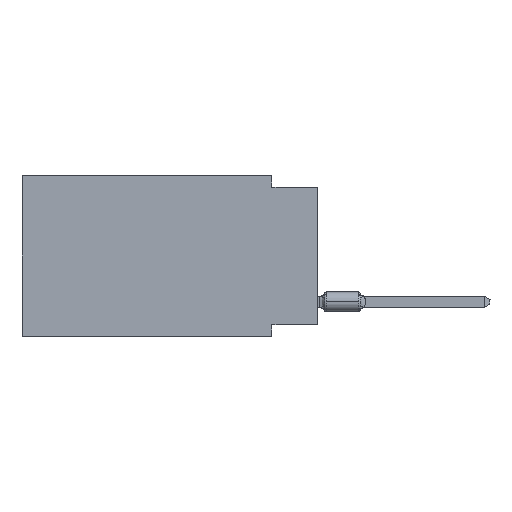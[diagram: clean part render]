
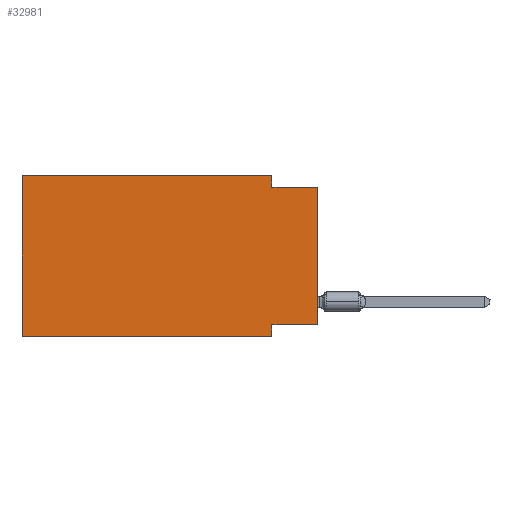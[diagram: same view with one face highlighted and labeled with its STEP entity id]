
A CAD part, left-side view. The second image highlights one B-rep face of the part: STEP entity #32981.
In plain terms, the highlighted planar face has unit normal (-1, 0, 0).
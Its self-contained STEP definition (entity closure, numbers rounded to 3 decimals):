
#937 = DIRECTION ( 'NONE',  ( 0., 0., -1. ) ) ;
#3139 = CARTESIAN_POINT ( 'NONE',  ( 0., 0., 0. ) ) ;
#5009 = DIRECTION ( 'NONE',  ( 0., 0., -1. ) ) ;
#5871 = ORIENTED_EDGE ( 'NONE', *, *, #47507, .F. ) ;
#8277 = EDGE_CURVE ( 'NONE', #50428, #93197, #84382, .T. ) ;
#11157 = ORIENTED_EDGE ( 'NONE', *, *, #21872, .F. ) ;
#12408 = DIRECTION ( 'NONE',  ( 0., 0., -1. ) ) ;
#14637 = DIRECTION ( 'NONE',  ( 0., 1., 0. ) ) ;
#19350 = ORIENTED_EDGE ( 'NONE', *, *, #37590, .F. ) ;
#19694 = DIRECTION ( 'NONE',  ( 0., 0., 1. ) ) ;
#21663 = CARTESIAN_POINT ( 'NONE',  ( 0., 2.54, -8.255 ) ) ;
#21872 = EDGE_CURVE ( 'NONE', #93706, #64156, #83534, .T. ) ;
#22099 = CARTESIAN_POINT ( 'NONE',  ( 0., 2.54, 0. ) ) ;
#23579 = CARTESIAN_POINT ( 'NONE',  ( 0., 16.383, 0. ) ) ;
#24098 = LINE ( 'NONE', #56725, #70165 ) ;
#24640 = CARTESIAN_POINT ( 'NONE',  ( 0., 16.383, -8.89 ) ) ;
#24644 = EDGE_CURVE ( 'NONE', #91051, #93197, #24098, .T. ) ;
#25724 = VECTOR ( 'NONE', #14637, 1000. ) ;
#25810 = EDGE_CURVE ( 'NONE', #64417, #26531, #81307, .T. ) ;
#26531 = VERTEX_POINT ( 'NONE', #54907 ) ;
#27731 = VECTOR ( 'NONE', #87739, 1000. ) ;
#29059 = LINE ( 'NONE', #22099, #90277 ) ;
#31753 = CARTESIAN_POINT ( 'NONE',  ( 0., 0., -8.255 ) ) ;
#32981 = ADVANCED_FACE ( 'NONE', ( #86282 ), #53676, .F. ) ;
#34753 = VERTEX_POINT ( 'NONE', #58322 ) ;
#37590 = EDGE_CURVE ( 'NONE', #50428, #93706, #55281, .T. ) ;
#40272 = VECTOR ( 'NONE', #19694, 1000. ) ;
#44098 = DIRECTION ( 'NONE',  ( 1., 0., 0. ) ) ;
#44999 = EDGE_CURVE ( 'NONE', #26531, #34753, #105078, .T. ) ;
#45669 = CARTESIAN_POINT ( 'NONE',  ( 0., 16.383, 0. ) ) ;
#46533 = CARTESIAN_POINT ( 'NONE',  ( 0., 2.54, -8.89 ) ) ;
#47507 = EDGE_CURVE ( 'NONE', #34753, #91051, #29059, .T. ) ;
#49177 = VECTOR ( 'NONE', #12408, 1000. ) ;
#50428 = VERTEX_POINT ( 'NONE', #71723 ) ;
#53676 = PLANE ( 'NONE',  #61185 ) ;
#54407 = CARTESIAN_POINT ( 'NONE',  ( 0., 0., -0.635 ) ) ;
#54907 = CARTESIAN_POINT ( 'NONE',  ( 0., 16.383, 0. ) ) ;
#55112 = EDGE_CURVE ( 'NONE', #64417, #64156, #89337, .T. ) ;
#55281 = LINE ( 'NONE', #31753, #25724 ) ;
#56725 = CARTESIAN_POINT ( 'NONE',  ( 0., 0., -0.635 ) ) ;
#58322 = CARTESIAN_POINT ( 'NONE',  ( 0., 2.54, 0. ) ) ;
#61089 = CARTESIAN_POINT ( 'NONE',  ( 0., 2.54, -0.635 ) ) ;
#61185 = AXIS2_PLACEMENT_3D ( 'NONE', #45669, #44098, #937 ) ;
#63545 = ORIENTED_EDGE ( 'NONE', *, *, #25810, .F. ) ;
#64156 = VERTEX_POINT ( 'NONE', #46533 ) ;
#64417 = VERTEX_POINT ( 'NONE', #71912 ) ;
#65800 = DIRECTION ( 'NONE',  ( 0., -1., 0. ) ) ;
#70165 = VECTOR ( 'NONE', #89311, 1000. ) ;
#71723 = CARTESIAN_POINT ( 'NONE',  ( 0., 0., -8.255 ) ) ;
#71912 = CARTESIAN_POINT ( 'NONE',  ( 0., 16.383, -8.89 ) ) ;
#78301 = EDGE_LOOP ( 'NONE', ( #78393, #88580, #5871, #92459, #63545, #98937, #11157, #19350 ) ) ;
#78393 = ORIENTED_EDGE ( 'NONE', *, *, #8277, .T. ) ;
#81028 = DIRECTION ( 'NONE',  ( 0., -1., 0. ) ) ;
#81307 = LINE ( 'NONE', #23579, #27731 ) ;
#83534 = LINE ( 'NONE', #99028, #49177 ) ;
#84382 = LINE ( 'NONE', #3139, #40272 ) ;
#86282 = FACE_OUTER_BOUND ( 'NONE', #78301, .T. ) ;
#87739 = DIRECTION ( 'NONE',  ( 0., 0., 1. ) ) ;
#88519 = CARTESIAN_POINT ( 'NONE',  ( 0., 16.383, 0. ) ) ;
#88580 = ORIENTED_EDGE ( 'NONE', *, *, #24644, .F. ) ;
#89311 = DIRECTION ( 'NONE',  ( 0., -1., 0. ) ) ;
#89337 = LINE ( 'NONE', #24640, #91374 ) ;
#90277 = VECTOR ( 'NONE', #5009, 1000. ) ;
#91051 = VERTEX_POINT ( 'NONE', #61089 ) ;
#91374 = VECTOR ( 'NONE', #65800, 1000. ) ;
#92459 = ORIENTED_EDGE ( 'NONE', *, *, #44999, .F. ) ;
#93197 = VERTEX_POINT ( 'NONE', #54407 ) ;
#93706 = VERTEX_POINT ( 'NONE', #21663 ) ;
#98937 = ORIENTED_EDGE ( 'NONE', *, *, #55112, .T. ) ;
#99028 = CARTESIAN_POINT ( 'NONE',  ( 0., 2.54, -8.89 ) ) ;
#101780 = VECTOR ( 'NONE', #81028, 1000. ) ;
#105078 = LINE ( 'NONE', #88519, #101780 ) ;
